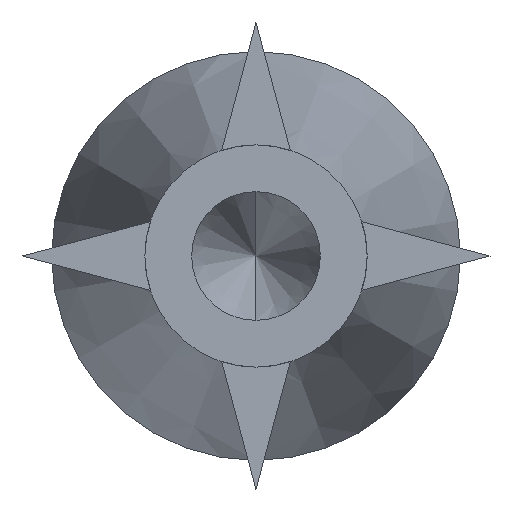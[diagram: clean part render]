
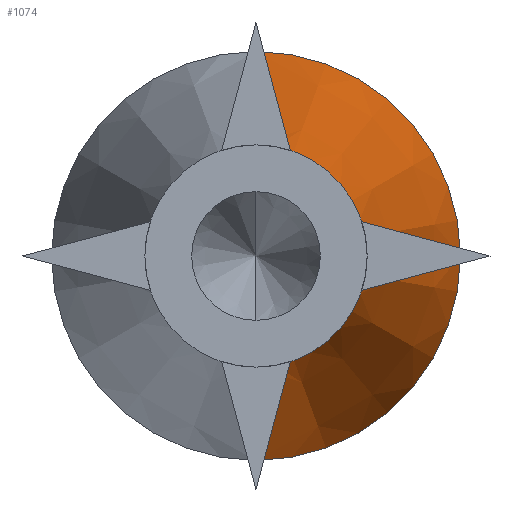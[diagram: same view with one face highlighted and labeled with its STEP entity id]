
A CAD part, front view. The second image highlights one B-rep face of the part: STEP entity #1074.
In plain terms, the highlighted conical face has half-angle 12.323 degrees and reference radius 19 mm.
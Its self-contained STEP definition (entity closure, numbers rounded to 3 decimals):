
#119 = ORIENTED_EDGE ( 'NONE', *, *, #1027, .F. ) ;
#134 = ORIENTED_EDGE ( 'NONE', *, *, #1022, .T. ) ;
#149 = ORIENTED_EDGE ( 'NONE', *, *, #1026, .T. ) ;
#150 = ORIENTED_EDGE ( 'NONE', *, *, #1033, .F. ) ;
#195 = VERTEX_POINT ( 'NONE', #404 ) ;
#196 = VERTEX_POINT ( 'NONE', #405 ) ;
#197 = VERTEX_POINT ( 'NONE', #406 ) ;
#223 = VERTEX_POINT ( 'NONE', #432 ) ;
#298 = EDGE_LOOP ( 'NONE', ( #119, #149, #134, #150 ) ) ;
#404 = CARTESIAN_POINT ( 'NONE',  ( 0., 182., -19. ) ) ;
#405 = CARTESIAN_POINT ( 'NONE',  ( 0., 255., -34.947 ) ) ;
#406 = CARTESIAN_POINT ( 'NONE',  ( 0., 182., 19. ) ) ;
#432 = CARTESIAN_POINT ( 'NONE',  ( 0., 255., 34.947 ) ) ;
#506 = CARTESIAN_POINT ( 'NONE',  ( 0., 255., 0. ) ) ;
#507 = DIRECTION ( 'NONE',  ( 0., -1., 0. ) ) ;
#508 = DIRECTION ( 'NONE',  ( 0., 0., -1. ) ) ;
#518 = CARTESIAN_POINT ( 'NONE',  ( 0., 182., 0. ) ) ;
#519 = LINE ( 'NONE', #520, #838 ) ;
#520 = CARTESIAN_POINT ( 'NONE',  ( 0., 182., -19. ) ) ;
#521 = DIRECTION ( 'NONE',  ( 0., 0.977, -0.213 ) ) ;
#522 = DIRECTION ( 'NONE',  ( 0., -1., 0. ) ) ;
#523 = DIRECTION ( 'NONE',  ( 0., 0., -1. ) ) ;
#540 = LINE ( 'NONE', #541, #846 ) ;
#541 = CARTESIAN_POINT ( 'NONE',  ( 0., 182., 19. ) ) ;
#542 = DIRECTION ( 'NONE',  ( 0., 0.977, 0.213 ) ) ;
#671 = CARTESIAN_POINT ( 'NONE',  ( 0., 182., 0. ) ) ;
#672 = DIRECTION ( 'NONE',  ( 0., 1., 0. ) ) ;
#673 = DIRECTION ( 'NONE',  ( 0., 0., 1. ) ) ;
#829 = AXIS2_PLACEMENT_3D ( 'NONE', #506, #507, #508 ) ;
#836 = AXIS2_PLACEMENT_3D ( 'NONE', #518, #522, #523 ) ;
#838 = VECTOR ( 'NONE', #521, 1000. ) ;
#846 = VECTOR ( 'NONE', #542, 1000. ) ;
#887 = FACE_OUTER_BOUND ( 'NONE', #298, .T. ) ;
#895 = AXIS2_PLACEMENT_3D ( 'NONE', #671, #672, #673 ) ;
#1022 = EDGE_CURVE ( 'NONE', #196, #223, #1136, .T. ) ;
#1026 = EDGE_CURVE ( 'NONE', #195, #196, #519, .T. ) ;
#1027 = EDGE_CURVE ( 'NONE', #195, #197, #1141, .T. ) ;
#1033 = EDGE_CURVE ( 'NONE', #197, #223, #540, .T. ) ;
#1074 = ADVANCED_FACE ( 'NONE', ( #887 ), #1167, .T. ) ;
#1136 = CIRCLE ( 'NONE', #829, 34.947 ) ;
#1141 = CIRCLE ( 'NONE', #836, 19. ) ;
#1167 = CONICAL_SURFACE ( 'NONE', #895, 19., 0.215 ) ;
